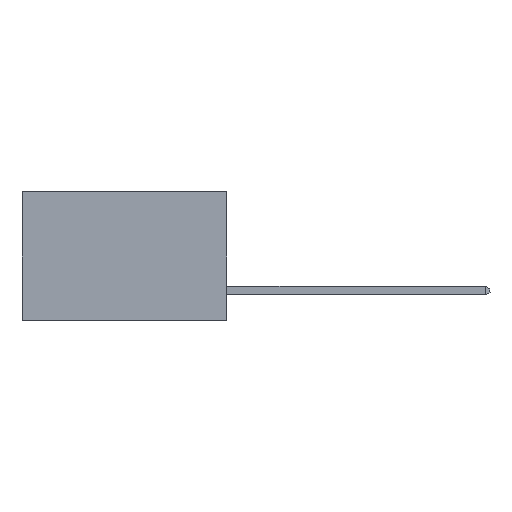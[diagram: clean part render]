
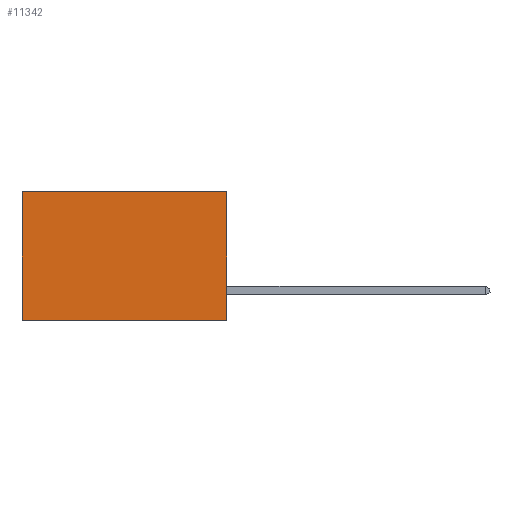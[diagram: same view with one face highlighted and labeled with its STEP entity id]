
A CAD part, left-side view. The second image highlights one B-rep face of the part: STEP entity #11342.
In plain terms, the highlighted planar face has unit normal (-1, 0, 0).
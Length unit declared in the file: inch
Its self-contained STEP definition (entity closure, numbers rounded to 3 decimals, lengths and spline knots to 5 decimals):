
#265 = EDGE_CURVE ( 'NONE', #15157, #10908, #1851, .T. ) ;
#274 = DIRECTION ( 'NONE',  ( 0., 0., -1. ) ) ;
#409 = LINE ( 'NONE', #9200, #6122 ) ;
#457 = VERTEX_POINT ( 'NONE', #14237 ) ;
#626 = EDGE_LOOP ( 'NONE', ( #11977, #9049, #12377, #6022 ) ) ;
#1814 = CARTESIAN_POINT ( 'NONE',  ( 0.277, 0.59, -0.37 ) ) ;
#1851 = LINE ( 'NONE', #6722, #2654 ) ;
#2369 = AXIS2_PLACEMENT_3D ( 'NONE', #15492, #8080, #274 ) ;
#2394 = VECTOR ( 'NONE', #5443, 39.37008 ) ;
#2654 = VECTOR ( 'NONE', #11850, 39.37008 ) ;
#5443 = DIRECTION ( 'NONE',  ( 0., 0., -1. ) ) ;
#5444 = CARTESIAN_POINT ( 'NONE',  ( 0.277, 0., -0.37 ) ) ;
#5859 = LINE ( 'NONE', #6655, #2394 ) ;
#6021 = EDGE_CURVE ( 'NONE', #13861, #15157, #409, .T. ) ;
#6022 = ORIENTED_EDGE ( 'NONE', *, *, #8478, .T. ) ;
#6122 = VECTOR ( 'NONE', #11105, 39.37008 ) ;
#6655 = CARTESIAN_POINT ( 'NONE',  ( 0.277, 0.59, -0.37 ) ) ;
#6722 = CARTESIAN_POINT ( 'NONE',  ( 0.277, 0., -0.37 ) ) ;
#6757 = PLANE ( 'NONE',  #2369 ) ;
#8080 = DIRECTION ( 'NONE',  ( 1., 0., 0. ) ) ;
#8178 = VECTOR ( 'NONE', #11923, 39.37008 ) ;
#8478 = EDGE_CURVE ( 'NONE', #13861, #457, #14013, .T. ) ;
#9049 = ORIENTED_EDGE ( 'NONE', *, *, #265, .F. ) ;
#9200 = CARTESIAN_POINT ( 'NONE',  ( 0.277, 0., -0.37 ) ) ;
#10908 = VERTEX_POINT ( 'NONE', #1814 ) ;
#11105 = DIRECTION ( 'NONE',  ( 0., 0., -1. ) ) ;
#11342 = ADVANCED_FACE ( 'NONE', ( #15641 ), #6757, .F. ) ;
#11850 = DIRECTION ( 'NONE',  ( 0., 1., 0. ) ) ;
#11923 = DIRECTION ( 'NONE',  ( 0., 1., 0. ) ) ;
#11957 = EDGE_CURVE ( 'NONE', #457, #10908, #5859, .T. ) ;
#11977 = ORIENTED_EDGE ( 'NONE', *, *, #11957, .T. ) ;
#11983 = CARTESIAN_POINT ( 'NONE',  ( 0.277, 0., 0. ) ) ;
#12377 = ORIENTED_EDGE ( 'NONE', *, *, #6021, .F. ) ;
#13861 = VERTEX_POINT ( 'NONE', #15405 ) ;
#14013 = LINE ( 'NONE', #11983, #8178 ) ;
#14237 = CARTESIAN_POINT ( 'NONE',  ( 0.277, 0.59, 0. ) ) ;
#15157 = VERTEX_POINT ( 'NONE', #5444 ) ;
#15405 = CARTESIAN_POINT ( 'NONE',  ( 0.277, 0., 0. ) ) ;
#15492 = CARTESIAN_POINT ( 'NONE',  ( 0.277, 0., -0.37 ) ) ;
#15641 = FACE_OUTER_BOUND ( 'NONE', #626, .T. ) ;
